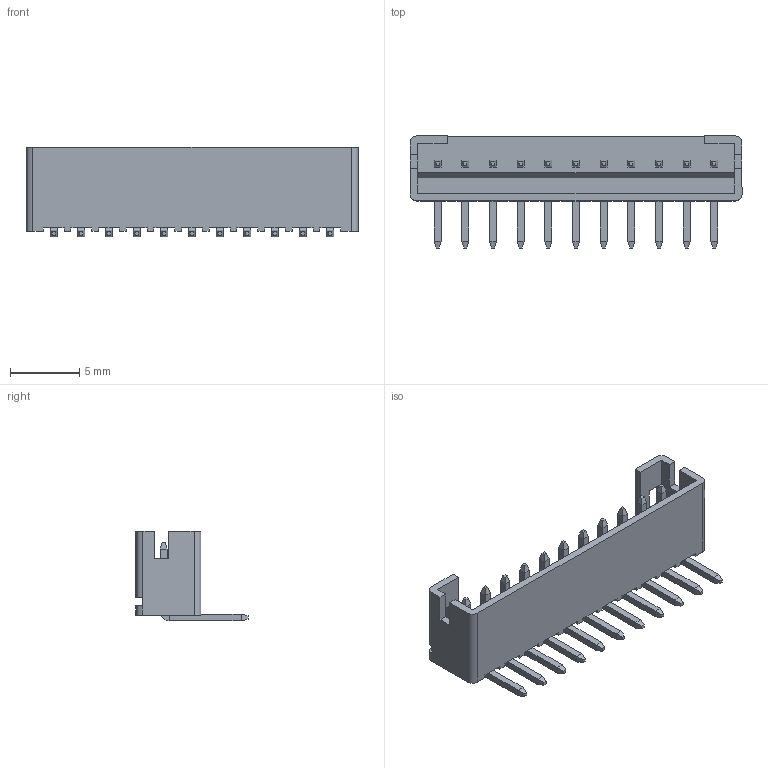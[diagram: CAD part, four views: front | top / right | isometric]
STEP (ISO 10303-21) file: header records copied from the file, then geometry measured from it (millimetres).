
FILE_DESCRIPTION (( 'STEP AP203' ), '1' );
FILE_NAME ('140-511-415-100.STEP', '2020-09-25T11:01:02', ( '' ), ( '' ), 'SwSTEP 2.0', 'SolidWorks 2020', '' );
FILE_SCHEMA (( 'CONFIG_CONTROL_DESIGN' ));
Length unit declared in the file: millimetre
Products named in the file (3): RA LI Contact_Str; RA LI Housing_511; 140-511-415-100
Assembly tree (12 placements, depth 2):
  140-511-415-100
    RA LI Housing_511
    RA LI Contact_Str  x11
Bounding box: 24 x 8.1 x 6.5 mm (x, y, z)
Volume: 258.6 mm3; surface area: 977 mm2
Topology: 12 solids, 12 shells, 370 faces, 864 edges, 516 vertices
Faces by surface type: plane 342, cylinder 28
Entity records: 5421 total; most frequent: CARTESIAN_POINT 865, ORIENTED_EDGE 848, DIRECTION 770, EDGE_CURVE 424, VECTOR 408, LINE 408, VERTEX_POINT 276, AXIS2_PLACEMENT_3D 181
